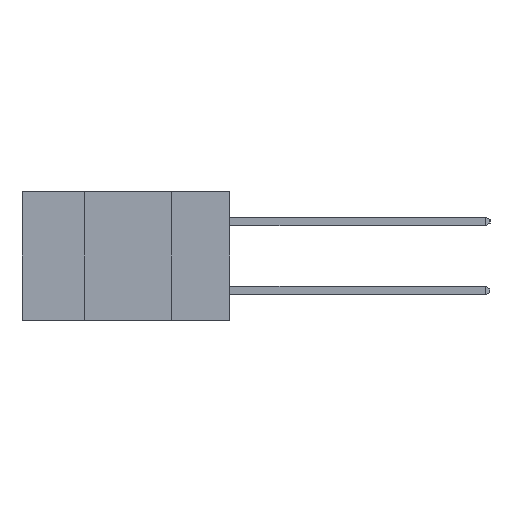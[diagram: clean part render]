
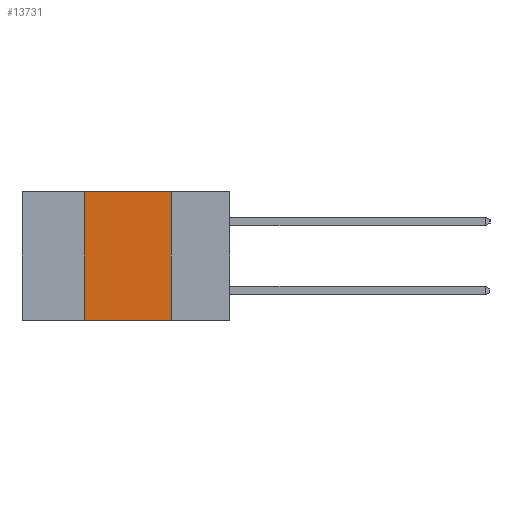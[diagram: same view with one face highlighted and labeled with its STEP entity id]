
A CAD part, left-side view. The second image highlights one B-rep face of the part: STEP entity #13731.
In plain terms, the highlighted planar face has unit normal (-1, 0, 0).
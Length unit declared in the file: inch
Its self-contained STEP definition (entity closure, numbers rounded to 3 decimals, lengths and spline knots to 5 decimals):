
#27 = CARTESIAN_POINT ( 'NONE',  ( 0., 0.17, 0. ) ) ;
#86 = EDGE_LOOP ( 'NONE', ( #7930, #2042, #7503, #6070 ) ) ;
#497 = DIRECTION ( 'NONE',  ( 0., -1., 0. ) ) ;
#1257 = LINE ( 'NONE', #27, #13288 ) ;
#1421 = DIRECTION ( 'NONE',  ( 0., 0., 1. ) ) ;
#2042 = ORIENTED_EDGE ( 'NONE', *, *, #11056, .F. ) ;
#2298 = LINE ( 'NONE', #12163, #5801 ) ;
#2944 = PLANE ( 'NONE',  #5041 ) ;
#4097 = DIRECTION ( 'NONE',  ( 0., 0., -1. ) ) ;
#4135 = VERTEX_POINT ( 'NONE', #10465 ) ;
#5041 = AXIS2_PLACEMENT_3D ( 'NONE', #6415, #11110, #4097 ) ;
#5331 = VECTOR ( 'NONE', #8569, 39.37008 ) ;
#5801 = VECTOR ( 'NONE', #497, 39.37008 ) ;
#5895 = CARTESIAN_POINT ( 'NONE',  ( 0., 0.6, -0.37 ) ) ;
#6070 = ORIENTED_EDGE ( 'NONE', *, *, #8020, .T. ) ;
#6414 = VERTEX_POINT ( 'NONE', #8972 ) ;
#6415 = CARTESIAN_POINT ( 'NONE',  ( 0., 0.6, 0. ) ) ;
#6962 = VECTOR ( 'NONE', #1421, 39.37008 ) ;
#7068 = DIRECTION ( 'NONE',  ( 0., 0., -1. ) ) ;
#7226 = EDGE_CURVE ( 'NONE', #11127, #6414, #10098, .T. ) ;
#7503 = ORIENTED_EDGE ( 'NONE', *, *, #7226, .F. ) ;
#7930 = ORIENTED_EDGE ( 'NONE', *, *, #13461, .F. ) ;
#8020 = EDGE_CURVE ( 'NONE', #11127, #4135, #11531, .T. ) ;
#8569 = DIRECTION ( 'NONE',  ( 0., -1., 0. ) ) ;
#8972 = CARTESIAN_POINT ( 'NONE',  ( 0., 0.42, 0. ) ) ;
#9301 = FACE_OUTER_BOUND ( 'NONE', #86, .T. ) ;
#9923 = CARTESIAN_POINT ( 'NONE',  ( 0., 0.17, 0. ) ) ;
#10098 = LINE ( 'NONE', #12537, #6962 ) ;
#10465 = CARTESIAN_POINT ( 'NONE',  ( 0., 0.17, -0.37 ) ) ;
#11056 = EDGE_CURVE ( 'NONE', #6414, #12506, #2298, .T. ) ;
#11110 = DIRECTION ( 'NONE',  ( 1., 0., 0. ) ) ;
#11127 = VERTEX_POINT ( 'NONE', #13444 ) ;
#11531 = LINE ( 'NONE', #5895, #5331 ) ;
#12163 = CARTESIAN_POINT ( 'NONE',  ( 0., 0.6, 0. ) ) ;
#12506 = VERTEX_POINT ( 'NONE', #9923 ) ;
#12537 = CARTESIAN_POINT ( 'NONE',  ( 0., 0.42, 0. ) ) ;
#13288 = VECTOR ( 'NONE', #7068, 39.37008 ) ;
#13444 = CARTESIAN_POINT ( 'NONE',  ( 0., 0.42, -0.37 ) ) ;
#13461 = EDGE_CURVE ( 'NONE', #12506, #4135, #1257, .T. ) ;
#13731 = ADVANCED_FACE ( 'NONE', ( #9301 ), #2944, .F. ) ;
